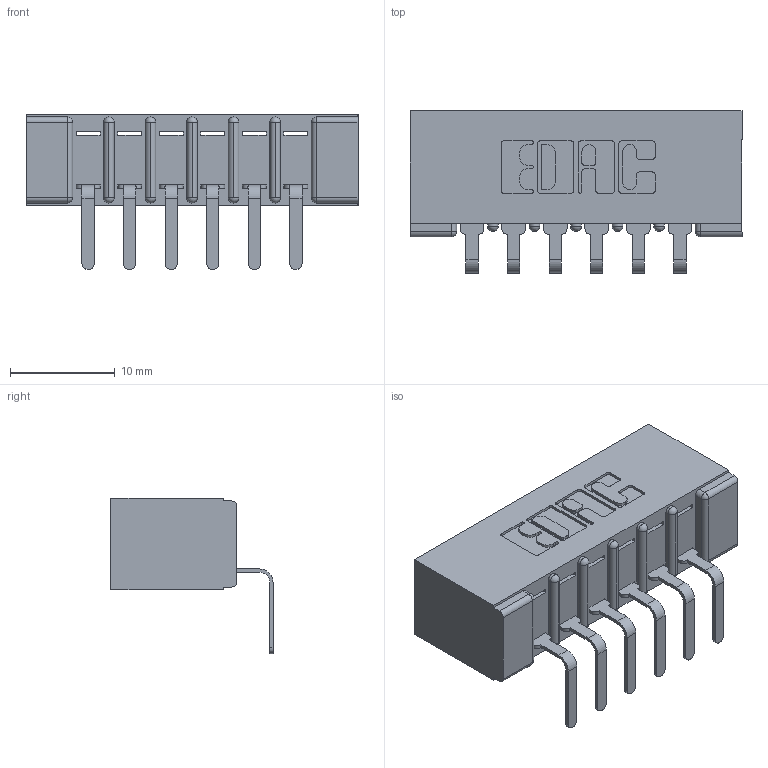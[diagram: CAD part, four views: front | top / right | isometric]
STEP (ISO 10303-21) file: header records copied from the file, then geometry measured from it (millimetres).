
FILE_DESCRIPTION (( 'STEP AP203' ), '1' );
FILE_NAME ('307-006-559-101.STEP', '2019-09-04T15:27:13', ( '' ), ( '' ), 'SwSTEP 2.0', 'SolidWorks 2016', '' );
FILE_SCHEMA (( 'CONFIG_CONTROL_DESIGN' ));
Length unit declared in the file: inch
Products named in the file (3): 307 Part_No Mounting Lugs; 307-290-001_558 559 - 1 (Single); 307-006-559-101
Assembly tree (7 placements, depth 2):
  307-006-559-101
    307 Part_No Mounting Lugs
    307-290-001_558 559 - 1 (Single)  x6
Bounding box: 31.65 x 15.46 x 14.81 mm (x, y, z)
Volume: 2244 mm3; surface area: 3231.1 mm2
Topology: 7 solids, 7 shells, 477 faces, 1343 edges, 866 vertices
Faces by surface type: plane 300, cylinder 163, sphere 14
Entity records: 9408 total; most frequent: CARTESIAN_POINT 1572, ORIENTED_EDGE 1558, DIRECTION 1549, EDGE_CURVE 779, LINE 583, VECTOR 583, VERTEX_POINT 506, AXIS2_PLACEMENT_3D 483
